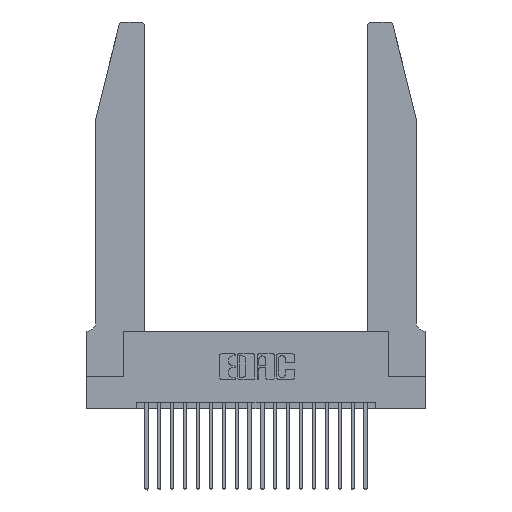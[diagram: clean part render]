
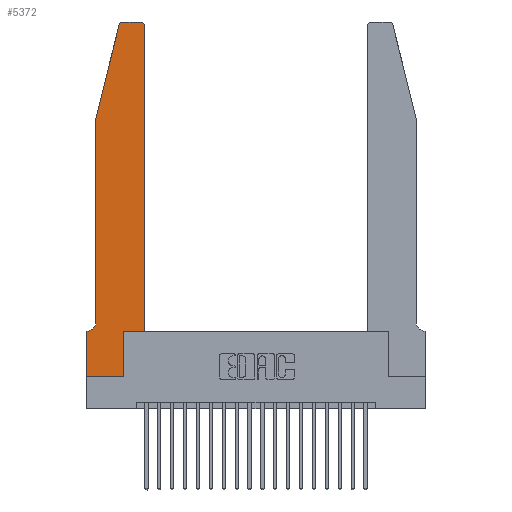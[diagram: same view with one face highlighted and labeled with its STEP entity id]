
A CAD part, top view. The second image highlights one B-rep face of the part: STEP entity #5372.
In plain terms, the highlighted planar face has unit normal (0, 0, 1).
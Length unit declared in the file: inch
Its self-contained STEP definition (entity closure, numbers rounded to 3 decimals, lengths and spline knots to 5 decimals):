
#172 = ORIENTED_EDGE ( 'NONE', *, *, #15323, .T. ) ;
#313 = VECTOR ( 'NONE', #8723, 39.37008 ) ;
#328 = VERTEX_POINT ( 'NONE', #12095 ) ;
#362 = EDGE_CURVE ( 'NONE', #6779, #15979, #11328, .T. ) ;
#369 = VERTEX_POINT ( 'NONE', #5574 ) ;
#409 = VERTEX_POINT ( 'NONE', #14235 ) ;
#889 = PLANE ( 'NONE',  #15832 ) ;
#940 = CARTESIAN_POINT ( 'NONE',  ( 0., 0., 0.37 ) ) ;
#1678 = DIRECTION ( 'NONE',  ( -1., 0., 0. ) ) ;
#2034 = DIRECTION ( 'NONE',  ( 0., 1., 0. ) ) ;
#2401 = DIRECTION ( 'NONE',  ( 0., 0., 1. ) ) ;
#2601 = DIRECTION ( 'NONE',  ( 1., 0., 0. ) ) ;
#2677 = CARTESIAN_POINT ( 'NONE',  ( 0.4205, 2.72, 0.37 ) ) ;
#3203 = VECTOR ( 'NONE', #2601, 39.37008 ) ;
#3766 = CIRCLE ( 'NONE', #22153, 0.03 ) ;
#4416 = ORIENTED_EDGE ( 'NONE', *, *, #17861, .T. ) ;
#4560 = CARTESIAN_POINT ( 'NONE',  ( 0.0755, 0.35, 0.37 ) ) ;
#4594 = VERTEX_POINT ( 'NONE', #11843 ) ;
#4599 = LINE ( 'NONE', #13080, #11300 ) ;
#5132 = ORIENTED_EDGE ( 'NONE', *, *, #18927, .T. ) ;
#5173 = CARTESIAN_POINT ( 'NONE',  ( 0.0755, 2., 0.37 ) ) ;
#5265 = EDGE_LOOP ( 'NONE', ( #172, #9294, #20284, #6706, #19968, #15771, #5132, #13823, #19979, #21903, #4416, #13494 ) ) ;
#5372 = ADVANCED_FACE ( 'NONE', ( #6600 ), #889, .T. ) ;
#5475 = CARTESIAN_POINT ( 'NONE',  ( 0.0055, 0.35, 0.37 ) ) ;
#5572 = CARTESIAN_POINT ( 'NONE',  ( 0.4505, 2.72, 0.37 ) ) ;
#5574 = CARTESIAN_POINT ( 'NONE',  ( 0.4205, 2.75, 0.37 ) ) ;
#5577 = CARTESIAN_POINT ( 'NONE',  ( 0.0755, 2., 0.37 ) ) ;
#5690 = DIRECTION ( 'NONE',  ( -1., 0., 0. ) ) ;
#6600 = FACE_OUTER_BOUND ( 'NONE', #5265, .T. ) ;
#6686 = LINE ( 'NONE', #4560, #18398 ) ;
#6706 = ORIENTED_EDGE ( 'NONE', *, *, #17055, .T. ) ;
#6779 = VERTEX_POINT ( 'NONE', #19493 ) ;
#6864 = EDGE_CURVE ( 'NONE', #12183, #15987, #21243, .T. ) ;
#7457 = VECTOR ( 'NONE', #20346, 39.37008 ) ;
#7589 = LINE ( 'NONE', #15508, #16148 ) ;
#7997 = CARTESIAN_POINT ( 'NONE',  ( 0., 0., 0.37 ) ) ;
#8213 = CARTESIAN_POINT ( 'NONE',  ( 0.284, 2.72, 0.37 ) ) ;
#8576 = VERTEX_POINT ( 'NONE', #940 ) ;
#8723 = DIRECTION ( 'NONE',  ( -0.239, -0.971, 0. ) ) ;
#9294 = ORIENTED_EDGE ( 'NONE', *, *, #17001, .T. ) ;
#9621 = VERTEX_POINT ( 'NONE', #14502 ) ;
#9625 = VECTOR ( 'NONE', #2034, 39.37008 ) ;
#9634 = DIRECTION ( 'NONE',  ( -1., 0., 0. ) ) ;
#9865 = AXIS2_PLACEMENT_3D ( 'NONE', #15912, #21203, #5690 ) ;
#10199 = VECTOR ( 'NONE', #17294, 39.37008 ) ;
#10582 = CARTESIAN_POINT ( 'NONE',  ( 0.4505, 0.35, 0.37 ) ) ;
#10965 = LINE ( 'NONE', #7997, #3203 ) ;
#11294 = DIRECTION ( 'NONE',  ( 1., 0., 0. ) ) ;
#11300 = VECTOR ( 'NONE', #11294, 39.37008 ) ;
#11328 = LINE ( 'NONE', #12256, #313 ) ;
#11524 = DIRECTION ( 'NONE',  ( 0., 0., 1. ) ) ;
#11843 = CARTESIAN_POINT ( 'NONE',  ( 0.2865, 0., 0.37 ) ) ;
#12095 = CARTESIAN_POINT ( 'NONE',  ( 0.2865, 0.35, 0.37 ) ) ;
#12183 = VERTEX_POINT ( 'NONE', #15184 ) ;
#12256 = CARTESIAN_POINT ( 'NONE',  ( 0.0755, 2., 0.37 ) ) ;
#12336 = EDGE_CURVE ( 'NONE', #15987, #409, #6686, .T. ) ;
#12532 = LINE ( 'NONE', #21921, #7457 ) ;
#12871 = CARTESIAN_POINT ( 'NONE',  ( 0., 0.35, 0.37 ) ) ;
#13080 = CARTESIAN_POINT ( 'NONE',  ( 0.4505, 0.35, 0.37 ) ) ;
#13494 = ORIENTED_EDGE ( 'NONE', *, *, #22145, .T. ) ;
#13730 = CARTESIAN_POINT ( 'NONE',  ( 0.2605, 2.75, 0.37 ) ) ;
#13740 = VECTOR ( 'NONE', #1678, 39.37008 ) ;
#13811 = DIRECTION ( 'NONE',  ( 1., 0., 0. ) ) ;
#13823 = ORIENTED_EDGE ( 'NONE', *, *, #17898, .T. ) ;
#14060 = VERTEX_POINT ( 'NONE', #21494 ) ;
#14235 = CARTESIAN_POINT ( 'NONE',  ( 0., 0.35, 0.37 ) ) ;
#14433 = CIRCLE ( 'NONE', #18213, 0.03 ) ;
#14502 = CARTESIAN_POINT ( 'NONE',  ( 0.4505, 0.35, 0.37 ) ) ;
#14548 = DIRECTION ( 'NONE',  ( 1., 0., 0. ) ) ;
#15036 = EDGE_CURVE ( 'NONE', #4594, #328, #7589, .T. ) ;
#15184 = CARTESIAN_POINT ( 'NONE',  ( 0.0755, 0.42, 0.37 ) ) ;
#15323 = EDGE_CURVE ( 'NONE', #369, #14060, #16408, .T. ) ;
#15508 = CARTESIAN_POINT ( 'NONE',  ( 0.2865, 0.35, 0.37 ) ) ;
#15563 = VERTEX_POINT ( 'NONE', #5572 ) ;
#15771 = ORIENTED_EDGE ( 'NONE', *, *, #12336, .T. ) ;
#15832 = AXIS2_PLACEMENT_3D ( 'NONE', #12871, #2401, #15977 ) ;
#15912 = CARTESIAN_POINT ( 'NONE',  ( 0.0055, 0.42, 0.37 ) ) ;
#15977 = DIRECTION ( 'NONE',  ( 1., 0., 0. ) ) ;
#15979 = VERTEX_POINT ( 'NONE', #5173 ) ;
#15987 = VERTEX_POINT ( 'NONE', #5475 ) ;
#16148 = VECTOR ( 'NONE', #17443, 39.37008 ) ;
#16408 = LINE ( 'NONE', #13730, #13740 ) ;
#16422 = DIRECTION ( 'NONE',  ( 0., 0., 1. ) ) ;
#16876 = EDGE_CURVE ( 'NONE', #328, #9621, #4599, .T. ) ;
#17001 = EDGE_CURVE ( 'NONE', #14060, #6779, #3766, .T. ) ;
#17055 = EDGE_CURVE ( 'NONE', #15979, #12183, #20065, .T. ) ;
#17294 = DIRECTION ( 'NONE',  ( 0., -1., 0. ) ) ;
#17443 = DIRECTION ( 'NONE',  ( 0., 1., 0. ) ) ;
#17861 = EDGE_CURVE ( 'NONE', #9621, #15563, #20298, .T. ) ;
#17898 = EDGE_CURVE ( 'NONE', #8576, #4594, #10965, .T. ) ;
#18213 = AXIS2_PLACEMENT_3D ( 'NONE', #2677, #16422, #14548 ) ;
#18398 = VECTOR ( 'NONE', #9634, 39.37008 ) ;
#18927 = EDGE_CURVE ( 'NONE', #409, #8576, #12532, .T. ) ;
#19493 = CARTESIAN_POINT ( 'NONE',  ( 0.25487, 2.72718, 0.37 ) ) ;
#19968 = ORIENTED_EDGE ( 'NONE', *, *, #6864, .T. ) ;
#19979 = ORIENTED_EDGE ( 'NONE', *, *, #15036, .T. ) ;
#20065 = LINE ( 'NONE', #5577, #10199 ) ;
#20284 = ORIENTED_EDGE ( 'NONE', *, *, #362, .T. ) ;
#20298 = LINE ( 'NONE', #10582, #9625 ) ;
#20346 = DIRECTION ( 'NONE',  ( 0., -1., 0. ) ) ;
#21203 = DIRECTION ( 'NONE',  ( 0., 0., -1. ) ) ;
#21243 = CIRCLE ( 'NONE', #9865, 0.07 ) ;
#21494 = CARTESIAN_POINT ( 'NONE',  ( 0.284, 2.75, 0.37 ) ) ;
#21903 = ORIENTED_EDGE ( 'NONE', *, *, #16876, .T. ) ;
#21921 = CARTESIAN_POINT ( 'NONE',  ( 0., 0., 0.37 ) ) ;
#22145 = EDGE_CURVE ( 'NONE', #15563, #369, #14433, .T. ) ;
#22153 = AXIS2_PLACEMENT_3D ( 'NONE', #8213, #11524, #13811 ) ;
